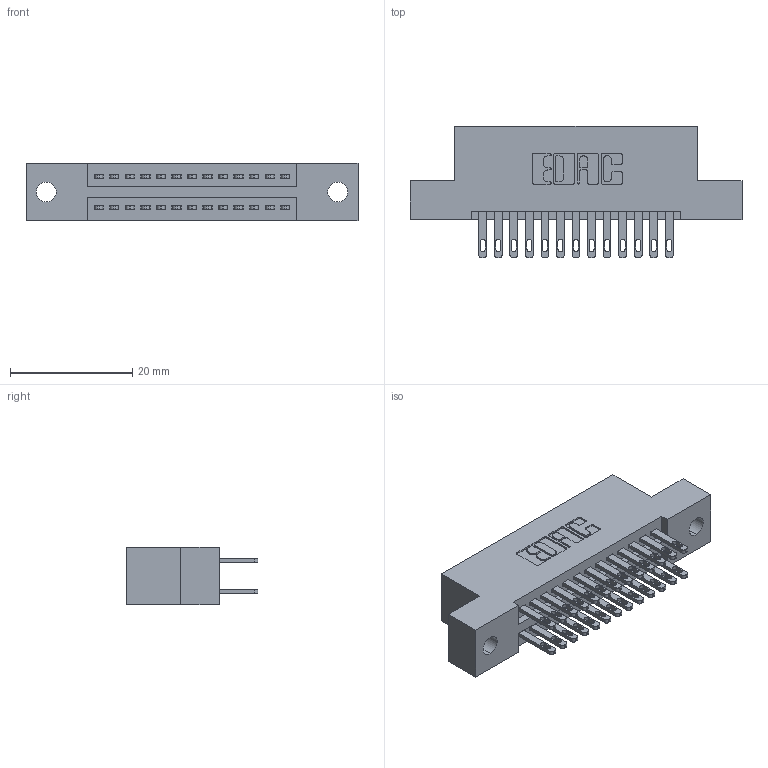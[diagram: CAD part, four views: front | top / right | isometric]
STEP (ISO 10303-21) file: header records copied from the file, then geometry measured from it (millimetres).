
FILE_DESCRIPTION (( 'STEP AP203' ), '1' );
FILE_NAME ('345-026-500-202.STEP', '2019-10-27T18:15:50', ( '' ), ( '' ), 'SwSTEP 2.0', 'SolidWorks 2016', '' );
FILE_SCHEMA (( 'CONFIG_CONTROL_DESIGN' ));
Length unit declared in the file: inch
Products named in the file (3): 345-292-001_345-293-100; 345 Part_Flush Mounting Lugs - 0.128 Dia; 345-026-500-202
Assembly tree (27 placements, depth 2):
  345-026-500-202
    345 Part_Flush Mounting Lugs - 0.128 Dia
    345-292-001_345-293-100  x26
Bounding box: 54.23 x 21.51 x 9.4 mm (x, y, z)
Volume: 5041.4 mm3; surface area: 6882.9 mm2
Topology: 27 solids, 27 shells, 1322 faces, 4007 edges, 2670 vertices
Faces by surface type: plane 782, cylinder 540
Entity records: 14037 total; most frequent: CARTESIAN_POINT 2380, ORIENTED_EDGE 2314, DIRECTION 2137, EDGE_CURVE 1157, VECTOR 969, LINE 969, VERTEX_POINT 770, AXIS2_PLACEMENT_3D 584
